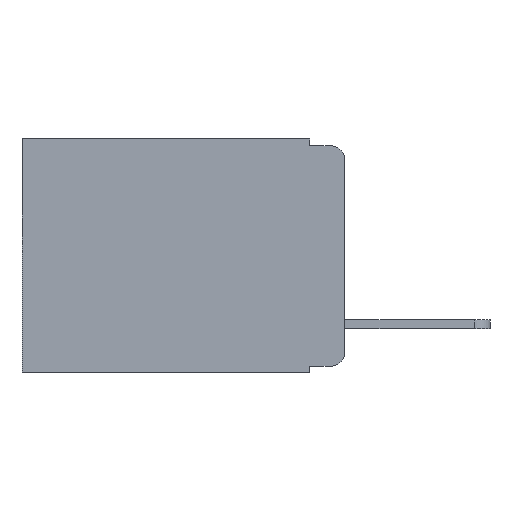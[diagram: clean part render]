
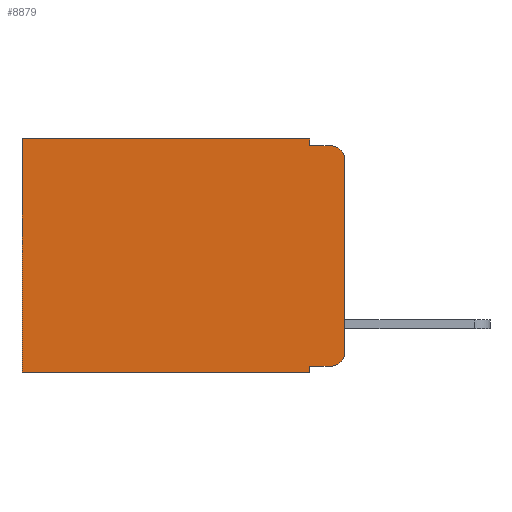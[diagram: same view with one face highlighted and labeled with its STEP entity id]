
A CAD part, left-side view. The second image highlights one B-rep face of the part: STEP entity #8879.
In plain terms, the highlighted planar face has unit normal (-1, 0, 0).
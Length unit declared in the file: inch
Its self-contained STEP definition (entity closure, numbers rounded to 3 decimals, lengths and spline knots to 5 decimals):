
#679 = ORIENTED_EDGE ( 'NONE', *, *, #10978, .F. ) ;
#1214 = EDGE_CURVE ( 'NONE', #16473, #8678, #10998, .T. ) ;
#1318 = VECTOR ( 'NONE', #14174, 39.37008 ) ;
#1472 = LINE ( 'NONE', #15120, #11406 ) ;
#1720 = PLANE ( 'NONE',  #7699 ) ;
#1738 = LINE ( 'NONE', #14924, #8615 ) ;
#1804 = DIRECTION ( 'NONE',  ( 0., -1., 0. ) ) ;
#2627 = ORIENTED_EDGE ( 'NONE', *, *, #12637, .F. ) ;
#2654 = ORIENTED_EDGE ( 'NONE', *, *, #6565, .F. ) ;
#2697 = VERTEX_POINT ( 'NONE', #17089 ) ;
#2811 = ORIENTED_EDGE ( 'NONE', *, *, #1214, .T. ) ;
#2827 = ORIENTED_EDGE ( 'NONE', *, *, #10135, .F. ) ;
#2857 = ORIENTED_EDGE ( 'NONE', *, *, #15964, .T. ) ;
#3170 = ORIENTED_EDGE ( 'NONE', *, *, #14310, .T. ) ;
#3212 = DIRECTION ( 'NONE',  ( 0., 0., -1. ) ) ;
#3490 = ORIENTED_EDGE ( 'NONE', *, *, #11822, .T. ) ;
#3762 = CARTESIAN_POINT ( 'NONE',  ( 0.298, 0., -0.343 ) ) ;
#3852 = LINE ( 'NONE', #6825, #10547 ) ;
#3910 = VECTOR ( 'NONE', #10991, 39.37008 ) ;
#4184 = CARTESIAN_POINT ( 'NONE',  ( 0.298, 0., -0.313 ) ) ;
#4595 = CARTESIAN_POINT ( 'NONE',  ( 0.298, 0.02, -0.333 ) ) ;
#4686 = ORIENTED_EDGE ( 'NONE', *, *, #16843, .F. ) ;
#4951 = CARTESIAN_POINT ( 'NONE',  ( 0.298, 0.02, -0.03 ) ) ;
#5806 = CARTESIAN_POINT ( 'NONE',  ( 0.298, 0.051, 0. ) ) ;
#5991 = EDGE_LOOP ( 'NONE', ( #2654, #13047, #2827, #679, #2811, #3490, #4686, #2627, #3170, #2857 ) ) ;
#6067 = CARTESIAN_POINT ( 'NONE',  ( 0.298, 0.02, -0.01 ) ) ;
#6151 = FACE_OUTER_BOUND ( 'NONE', #5991, .T. ) ;
#6301 = DIRECTION ( 'NONE',  ( 0., 0., -1. ) ) ;
#6565 = EDGE_CURVE ( 'NONE', #2697, #6635, #3852, .T. ) ;
#6612 = CIRCLE ( 'NONE', #12306, 0.02 ) ;
#6635 = VERTEX_POINT ( 'NONE', #4184 ) ;
#6825 = CARTESIAN_POINT ( 'NONE',  ( 0.298, 0., 0. ) ) ;
#6914 = VERTEX_POINT ( 'NONE', #12539 ) ;
#7577 = CARTESIAN_POINT ( 'NONE',  ( 0.298, 0.02, -0.313 ) ) ;
#7699 = AXIS2_PLACEMENT_3D ( 'NONE', #14858, #11162, #3212 ) ;
#8203 = DIRECTION ( 'NONE',  ( 0., 0., -1. ) ) ;
#8357 = EDGE_CURVE ( 'NONE', #2697, #15900, #8452, .T. ) ;
#8452 = CIRCLE ( 'NONE', #9257, 0.02 ) ;
#8615 = VECTOR ( 'NONE', #1804, 39.37008 ) ;
#8678 = VERTEX_POINT ( 'NONE', #12056 ) ;
#8879 = ADVANCED_FACE ( 'NONE', ( #6151 ), #1720, .F. ) ;
#8913 = DIRECTION ( 'NONE',  ( 0., 0., -1. ) ) ;
#9257 = AXIS2_PLACEMENT_3D ( 'NONE', #4951, #13990, #6301 ) ;
#9562 = CARTESIAN_POINT ( 'NONE',  ( 0.298, 0.051, -0.343 ) ) ;
#9729 = CARTESIAN_POINT ( 'NONE',  ( 0.298, 0.051, -0.333 ) ) ;
#10135 = EDGE_CURVE ( 'NONE', #6914, #15900, #1738, .T. ) ;
#10455 = VECTOR ( 'NONE', #13037, 39.37008 ) ;
#10547 = VECTOR ( 'NONE', #8203, 39.37008 ) ;
#10791 = VERTEX_POINT ( 'NONE', #14848 ) ;
#10978 = EDGE_CURVE ( 'NONE', #16473, #6914, #1472, .T. ) ;
#10991 = DIRECTION ( 'NONE',  ( 0., -1., 0. ) ) ;
#10998 = LINE ( 'NONE', #16171, #14304 ) ;
#11162 = DIRECTION ( 'NONE',  ( 1., 0., 0. ) ) ;
#11406 = VECTOR ( 'NONE', #16357, 39.37008 ) ;
#11421 = VECTOR ( 'NONE', #13750, 39.37008 ) ;
#11513 = VERTEX_POINT ( 'NONE', #4595 ) ;
#11822 = EDGE_CURVE ( 'NONE', #8678, #13362, #17046, .T. ) ;
#11824 = LINE ( 'NONE', #12296, #11421 ) ;
#12056 = CARTESIAN_POINT ( 'NONE',  ( 0.298, 0.473, 0. ) ) ;
#12088 = LINE ( 'NONE', #3762, #1318 ) ;
#12296 = CARTESIAN_POINT ( 'NONE',  ( 0.298, 0.051, 0. ) ) ;
#12306 = AXIS2_PLACEMENT_3D ( 'NONE', #7577, #16432, #8913 ) ;
#12539 = CARTESIAN_POINT ( 'NONE',  ( 0.298, 0.051, -0.01 ) ) ;
#12637 = EDGE_CURVE ( 'NONE', #10791, #14233, #11824, .T. ) ;
#13037 = DIRECTION ( 'NONE',  ( 0., 0., -1. ) ) ;
#13047 = ORIENTED_EDGE ( 'NONE', *, *, #8357, .T. ) ;
#13362 = VERTEX_POINT ( 'NONE', #14394 ) ;
#13750 = DIRECTION ( 'NONE',  ( 0., 0., -1. ) ) ;
#13990 = DIRECTION ( 'NONE',  ( -1., 0., 0. ) ) ;
#14153 = DIRECTION ( 'NONE',  ( 0., 1., 0. ) ) ;
#14174 = DIRECTION ( 'NONE',  ( 0., 1., 0. ) ) ;
#14233 = VERTEX_POINT ( 'NONE', #9562 ) ;
#14276 = CARTESIAN_POINT ( 'NONE',  ( 0.298, 0.473, 0. ) ) ;
#14288 = LINE ( 'NONE', #9729, #3910 ) ;
#14304 = VECTOR ( 'NONE', #14153, 39.37008 ) ;
#14310 = EDGE_CURVE ( 'NONE', #10791, #11513, #14288, .T. ) ;
#14394 = CARTESIAN_POINT ( 'NONE',  ( 0.298, 0.473, -0.343 ) ) ;
#14848 = CARTESIAN_POINT ( 'NONE',  ( 0.298, 0.051, -0.333 ) ) ;
#14858 = CARTESIAN_POINT ( 'NONE',  ( 0.298, 0., 0. ) ) ;
#14924 = CARTESIAN_POINT ( 'NONE',  ( 0.298, 0.051, -0.01 ) ) ;
#15120 = CARTESIAN_POINT ( 'NONE',  ( 0.298, 0.051, 0. ) ) ;
#15900 = VERTEX_POINT ( 'NONE', #6067 ) ;
#15964 = EDGE_CURVE ( 'NONE', #11513, #6635, #6612, .T. ) ;
#16171 = CARTESIAN_POINT ( 'NONE',  ( 0.298, 0., 0. ) ) ;
#16357 = DIRECTION ( 'NONE',  ( 0., 0., -1. ) ) ;
#16432 = DIRECTION ( 'NONE',  ( -1., 0., 0. ) ) ;
#16473 = VERTEX_POINT ( 'NONE', #5806 ) ;
#16843 = EDGE_CURVE ( 'NONE', #14233, #13362, #12088, .T. ) ;
#17046 = LINE ( 'NONE', #14276, #10455 ) ;
#17089 = CARTESIAN_POINT ( 'NONE',  ( 0.298, 0., -0.03 ) ) ;
